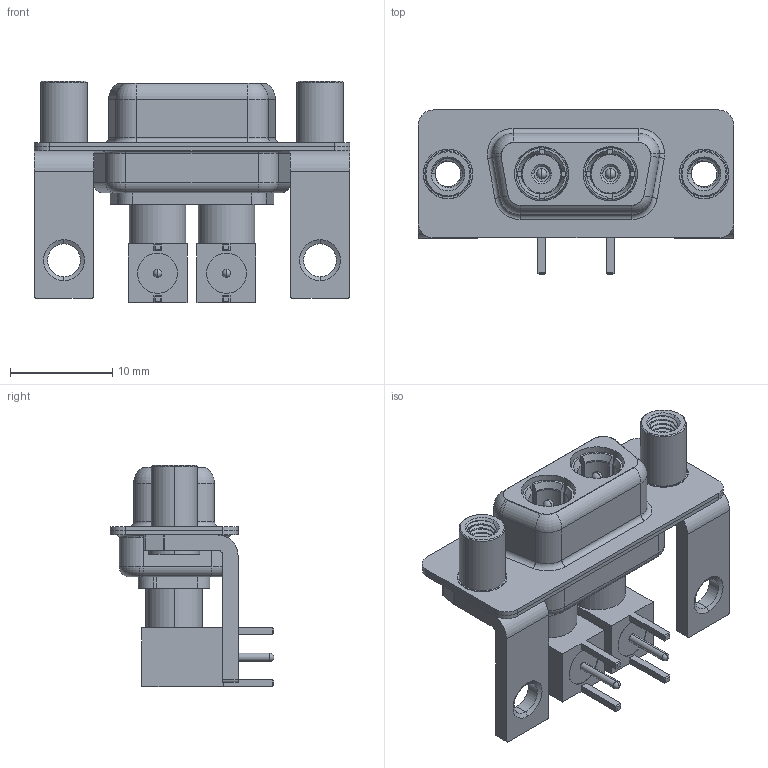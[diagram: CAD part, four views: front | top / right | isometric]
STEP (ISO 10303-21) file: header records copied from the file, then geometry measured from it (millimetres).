
FILE_DESCRIPTION (( 'STEP AP203' ), '1' );
FILE_NAME ('630-2W2-640-7TE.STEP', '2022-05-26T20:06:45', ( '' ), ( '' ), 'SwSTEP 2.0', 'SolidWorks 2020', '' );
FILE_SCHEMA (( 'CONFIG_CONTROL_DESIGN' ));
Length unit declared in the file: millimetre
Products named in the file (14): Co-Ax Plug Assy_RA; 630Combo Stabilizer Bracket; 630Combo Shell Front_09 Contacts; Locking Collar; Co-Ax Plug_RA PC Tail; 630Combo Housing_2W2; Insulator Pin_Straight PC Tail; 630-2W2-640-7TE; 630Combo Threaded Standoff_D; Pin_RA; Insulator RA Pin; 630Combo Shell Rear_09 Contacts; RA Back Shell
Assembly tree (21 placements, depth 3):
  630-2W2-640-7TE
    630Combo Housing_2W2
    630Combo Shell Front_09 Contacts
    630Combo Shell Rear_09 Contacts
    630Combo Stabilizer Bracket  x2
    630Combo Threaded Standoff_D  x2
    Co-Ax Plug Assy_RA
      Co-Ax Plug_RA PC Tail
      Insulator Pin_Straight PC Tail
      Pin_RA
      Locking Collar
      RA Back Shell
      Insulator RA Pin
    Co-Ax Plug Assy_RA
      Co-Ax Plug_RA PC Tail
      Insulator Pin_Straight PC Tail
      Pin_RA
      Locking Collar
      RA Back Shell
      Insulator RA Pin
Bounding box: 30.8 x 16 x 21.61 mm (x, y, z)
Volume: 2521.7 mm3; surface area: 6560.9 mm2
Topology: 19 solids, 19 shells, 713 faces, 1757 edges, 1107 vertices
Faces by surface type: cylinder 339, plane 223, torus 69, cone 66, bspline 8, sphere 8
Entity records: 17973 total; most frequent: CARTESIAN_POINT 5112, DIRECTION 2468, ORIENTED_EDGE 2280, EDGE_CURVE 1140, AXIS2_PLACEMENT_3D 984, VERTEX_POINT 721, EDGE_LOOP 525, VECTOR 500
